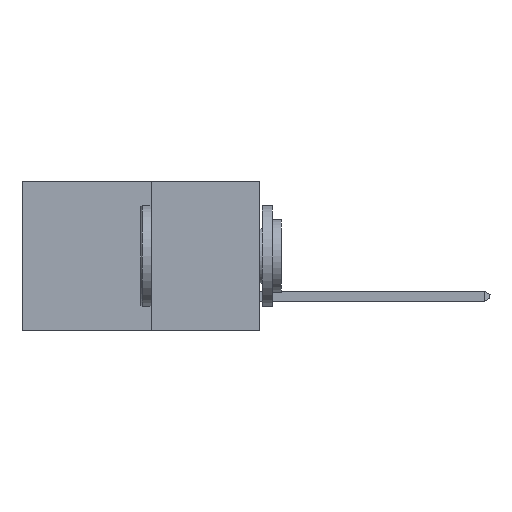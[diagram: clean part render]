
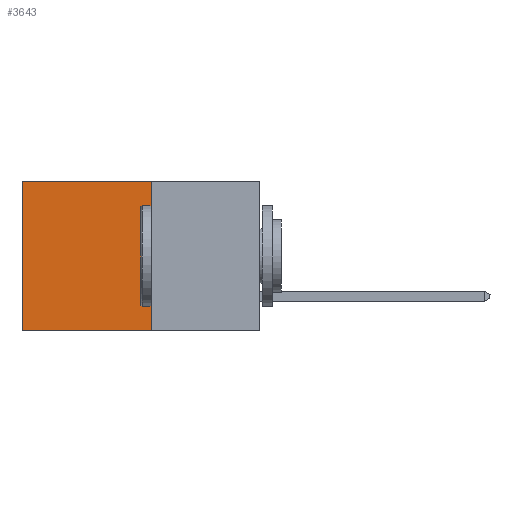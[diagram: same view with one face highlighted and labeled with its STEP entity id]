
A CAD part, left-side view. The second image highlights one B-rep face of the part: STEP entity #3643.
In plain terms, the highlighted planar face has unit normal (-1, 0, 0).
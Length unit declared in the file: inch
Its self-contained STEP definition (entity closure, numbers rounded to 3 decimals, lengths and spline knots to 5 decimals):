
#20 = DIRECTION ( 'NONE',  ( 0., 0., -1. ) ) ;
#69 = CARTESIAN_POINT ( 'NONE',  ( 0.277, 0.27, -0.37 ) ) ;
#740 = EDGE_LOOP ( 'NONE', ( #7807, #7323, #7630, #7351 ) ) ;
#755 = DIRECTION ( 'NONE',  ( 0., 0., -1. ) ) ;
#765 = CARTESIAN_POINT ( 'NONE',  ( 0.277, 0.27, -0.37 ) ) ;
#808 = EDGE_CURVE ( 'NONE', #6660, #7556, #7406, .T. ) ;
#1436 = EDGE_CURVE ( 'NONE', #7556, #6901, #8877, .T. ) ;
#3339 = LINE ( 'NONE', #69, #6877 ) ;
#3643 = ADVANCED_FACE ( 'NONE', ( #5166 ), #8567, .F. ) ;
#4925 = CARTESIAN_POINT ( 'NONE',  ( 0.277, 0.27, -0.37 ) ) ;
#5166 = FACE_OUTER_BOUND ( 'NONE', #740, .T. ) ;
#5304 = AXIS2_PLACEMENT_3D ( 'NONE', #7039, #7366, #755 ) ;
#5329 = CARTESIAN_POINT ( 'NONE',  ( 0.277, 0.59, -0.37 ) ) ;
#5517 = DIRECTION ( 'NONE',  ( 0., 1., 0. ) ) ;
#5653 = VECTOR ( 'NONE', #7073, 39.37008 ) ;
#5693 = LINE ( 'NONE', #4925, #7530 ) ;
#5958 = EDGE_CURVE ( 'NONE', #8604, #6901, #5693, .T. ) ;
#6270 = CARTESIAN_POINT ( 'NONE',  ( 0.277, 0.27, 0. ) ) ;
#6568 = DIRECTION ( 'NONE',  ( 0., 0., -1. ) ) ;
#6660 = VERTEX_POINT ( 'NONE', #8754 ) ;
#6877 = VECTOR ( 'NONE', #20, 39.37008 ) ;
#6901 = VERTEX_POINT ( 'NONE', #7464 ) ;
#7039 = CARTESIAN_POINT ( 'NONE',  ( 0.277, 0.27, -0.37 ) ) ;
#7065 = EDGE_CURVE ( 'NONE', #6660, #8604, #3339, .T. ) ;
#7073 = DIRECTION ( 'NONE',  ( 0., 1., 0. ) ) ;
#7323 = ORIENTED_EDGE ( 'NONE', *, *, #5958, .F. ) ;
#7351 = ORIENTED_EDGE ( 'NONE', *, *, #808, .T. ) ;
#7366 = DIRECTION ( 'NONE',  ( 1., 0., 0. ) ) ;
#7406 = LINE ( 'NONE', #6270, #5653 ) ;
#7464 = CARTESIAN_POINT ( 'NONE',  ( 0.277, 0.59, -0.37 ) ) ;
#7530 = VECTOR ( 'NONE', #5517, 39.37008 ) ;
#7556 = VERTEX_POINT ( 'NONE', #8343 ) ;
#7630 = ORIENTED_EDGE ( 'NONE', *, *, #7065, .F. ) ;
#7807 = ORIENTED_EDGE ( 'NONE', *, *, #1436, .T. ) ;
#8343 = CARTESIAN_POINT ( 'NONE',  ( 0.277, 0.59, 0. ) ) ;
#8567 = PLANE ( 'NONE',  #5304 ) ;
#8604 = VERTEX_POINT ( 'NONE', #765 ) ;
#8714 = VECTOR ( 'NONE', #6568, 39.37008 ) ;
#8754 = CARTESIAN_POINT ( 'NONE',  ( 0.277, 0.27, 0. ) ) ;
#8877 = LINE ( 'NONE', #5329, #8714 ) ;
